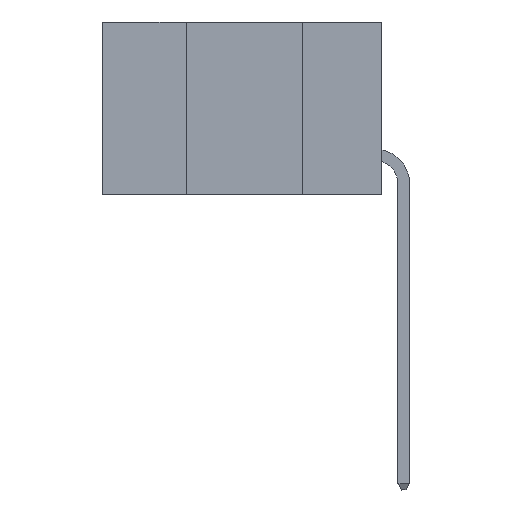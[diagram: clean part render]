
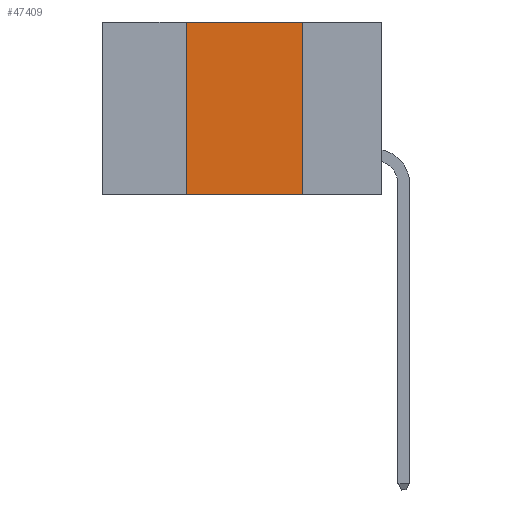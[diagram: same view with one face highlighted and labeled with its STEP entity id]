
A CAD part, left-side view. The second image highlights one B-rep face of the part: STEP entity #47409.
In plain terms, the highlighted planar face has unit normal (-1, 0, 0).
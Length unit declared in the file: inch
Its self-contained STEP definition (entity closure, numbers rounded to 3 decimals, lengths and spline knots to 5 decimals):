
#2482 = ORIENTED_EDGE ( 'NONE', *, *, #45208, .F. ) ;
#2511 = VERTEX_POINT ( 'NONE', #14717 ) ;
#2697 = LINE ( 'NONE', #32774, #28097 ) ;
#4179 = VERTEX_POINT ( 'NONE', #22169 ) ;
#7246 = FACE_OUTER_BOUND ( 'NONE', #9256, .T. ) ;
#7902 = EDGE_CURVE ( 'NONE', #2511, #31980, #37378, .T. ) ;
#9235 = VECTOR ( 'NONE', #31882, 39.37008 ) ;
#9256 = EDGE_LOOP ( 'NONE', ( #2482, #21583, #36440, #12166 ) ) ;
#10336 = CARTESIAN_POINT ( 'NONE',  ( 0., 0.42, 0. ) ) ;
#12166 = ORIENTED_EDGE ( 'NONE', *, *, #13977, .T. ) ;
#13977 = EDGE_CURVE ( 'NONE', #2511, #46738, #33025, .T. ) ;
#14323 = DIRECTION ( 'NONE',  ( 0., -1., 0. ) ) ;
#14717 = CARTESIAN_POINT ( 'NONE',  ( 0., 0.42, -0.37 ) ) ;
#15400 = VECTOR ( 'NONE', #27771, 39.37008 ) ;
#16219 = DIRECTION ( 'NONE',  ( 0., 0., -1. ) ) ;
#16230 = CARTESIAN_POINT ( 'NONE',  ( 0., 0.42, 0. ) ) ;
#16310 = DIRECTION ( 'NONE',  ( 0., 0., -1. ) ) ;
#18572 = EDGE_CURVE ( 'NONE', #31980, #4179, #2697, .T. ) ;
#21583 = ORIENTED_EDGE ( 'NONE', *, *, #18572, .F. ) ;
#22169 = CARTESIAN_POINT ( 'NONE',  ( 0., 0.17, 0. ) ) ;
#22993 = LINE ( 'NONE', #33976, #46818 ) ;
#27771 = DIRECTION ( 'NONE',  ( 0., 0., 1. ) ) ;
#28097 = VECTOR ( 'NONE', #14323, 39.37008 ) ;
#30829 = CARTESIAN_POINT ( 'NONE',  ( 0., 0.6, 0. ) ) ;
#31882 = DIRECTION ( 'NONE',  ( 0., -1., 0. ) ) ;
#31980 = VERTEX_POINT ( 'NONE', #10336 ) ;
#32774 = CARTESIAN_POINT ( 'NONE',  ( 0., 0.6, 0. ) ) ;
#33025 = LINE ( 'NONE', #42501, #9235 ) ;
#33976 = CARTESIAN_POINT ( 'NONE',  ( 0., 0.17, 0. ) ) ;
#36440 = ORIENTED_EDGE ( 'NONE', *, *, #7902, .F. ) ;
#37378 = LINE ( 'NONE', #16230, #15400 ) ;
#37894 = DIRECTION ( 'NONE',  ( 1., 0., 0. ) ) ;
#38596 = CARTESIAN_POINT ( 'NONE',  ( 0., 0.17, -0.37 ) ) ;
#40790 = AXIS2_PLACEMENT_3D ( 'NONE', #30829, #37894, #16219 ) ;
#42501 = CARTESIAN_POINT ( 'NONE',  ( 0., 0.6, -0.37 ) ) ;
#45208 = EDGE_CURVE ( 'NONE', #4179, #46738, #22993, .T. ) ;
#45687 = PLANE ( 'NONE',  #40790 ) ;
#46738 = VERTEX_POINT ( 'NONE', #38596 ) ;
#46818 = VECTOR ( 'NONE', #16310, 39.37008 ) ;
#47409 = ADVANCED_FACE ( 'NONE', ( #7246 ), #45687, .F. ) ;
